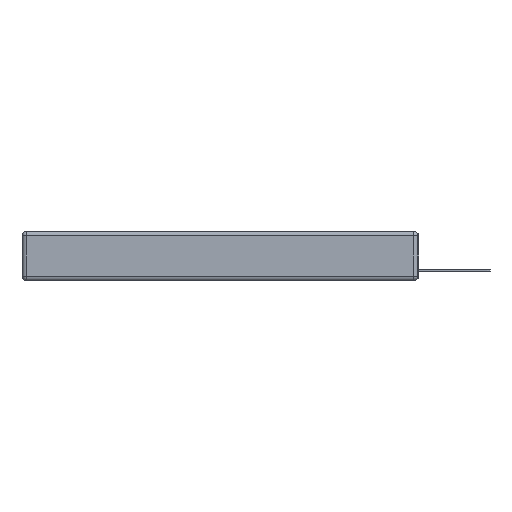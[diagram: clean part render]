
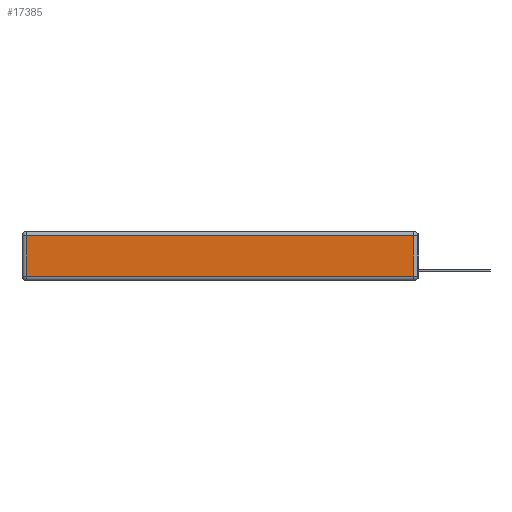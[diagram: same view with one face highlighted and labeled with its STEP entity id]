
A CAD part, left-side view. The second image highlights one B-rep face of the part: STEP entity #17385.
In plain terms, the highlighted planar face has unit normal (-1, 0, 0).
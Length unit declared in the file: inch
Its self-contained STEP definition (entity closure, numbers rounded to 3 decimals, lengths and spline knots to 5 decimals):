
#340 = EDGE_CURVE ( 'NONE', #5954, #5799, #7916, .T. ) ;
#414 = VERTEX_POINT ( 'NONE', #15016 ) ;
#1543 = VECTOR ( 'NONE', #13705, 39.37008 ) ;
#3209 = CARTESIAN_POINT ( 'NONE',  ( 0., 0., -0.343 ) ) ;
#4649 = CARTESIAN_POINT ( 'NONE',  ( 0., 2.72, -0.03 ) ) ;
#4880 = EDGE_LOOP ( 'NONE', ( #12072, #14589, #12149, #8796 ) ) ;
#5053 = VERTEX_POINT ( 'NONE', #4649 ) ;
#5304 = AXIS2_PLACEMENT_3D ( 'NONE', #3209, #14279, #9329 ) ;
#5496 = CARTESIAN_POINT ( 'NONE',  ( 0., 0.03, -0.03 ) ) ;
#5799 = VERTEX_POINT ( 'NONE', #5496 ) ;
#5954 = VERTEX_POINT ( 'NONE', #7311 ) ;
#6699 = VECTOR ( 'NONE', #11945, 39.37008 ) ;
#7311 = CARTESIAN_POINT ( 'NONE',  ( 0., 0.03, -0.313 ) ) ;
#7916 = LINE ( 'NONE', #9812, #8923 ) ;
#8392 = VECTOR ( 'NONE', #13898, 39.37008 ) ;
#8796 = ORIENTED_EDGE ( 'NONE', *, *, #17694, .T. ) ;
#8923 = VECTOR ( 'NONE', #13123, 39.37008 ) ;
#9016 = LINE ( 'NONE', #16964, #1543 ) ;
#9329 = DIRECTION ( 'NONE',  ( 0., 0., 1. ) ) ;
#9812 = CARTESIAN_POINT ( 'NONE',  ( 0., 0.03, -0.343 ) ) ;
#10864 = LINE ( 'NONE', #14077, #8392 ) ;
#10903 = EDGE_CURVE ( 'NONE', #5799, #5053, #10864, .T. ) ;
#10986 = PLANE ( 'NONE',  #5304 ) ;
#11945 = DIRECTION ( 'NONE',  ( 0., 0., -1. ) ) ;
#12072 = ORIENTED_EDGE ( 'NONE', *, *, #15391, .T. ) ;
#12149 = ORIENTED_EDGE ( 'NONE', *, *, #10903, .T. ) ;
#13123 = DIRECTION ( 'NONE',  ( 0., 0., 1. ) ) ;
#13705 = DIRECTION ( 'NONE',  ( 0., -1., 0. ) ) ;
#13898 = DIRECTION ( 'NONE',  ( 0., 1., 0. ) ) ;
#14077 = CARTESIAN_POINT ( 'NONE',  ( 0., 2.75, -0.03 ) ) ;
#14279 = DIRECTION ( 'NONE',  ( -1., 0., 0. ) ) ;
#14589 = ORIENTED_EDGE ( 'NONE', *, *, #340, .T. ) ;
#15016 = CARTESIAN_POINT ( 'NONE',  ( 0., 2.72, -0.313 ) ) ;
#15146 = CARTESIAN_POINT ( 'NONE',  ( 0., 2.72, -0.343 ) ) ;
#15391 = EDGE_CURVE ( 'NONE', #414, #5954, #9016, .T. ) ;
#15830 = FACE_OUTER_BOUND ( 'NONE', #4880, .T. ) ;
#16547 = LINE ( 'NONE', #15146, #6699 ) ;
#16964 = CARTESIAN_POINT ( 'NONE',  ( 0., 0., -0.313 ) ) ;
#17385 = ADVANCED_FACE ( 'NONE', ( #15830 ), #10986, .T. ) ;
#17694 = EDGE_CURVE ( 'NONE', #5053, #414, #16547, .T. ) ;
